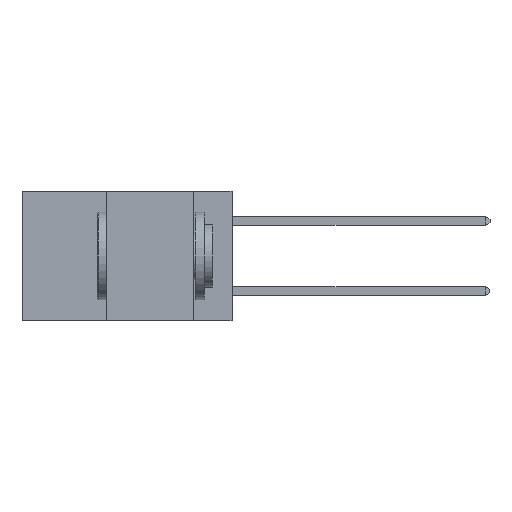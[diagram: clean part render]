
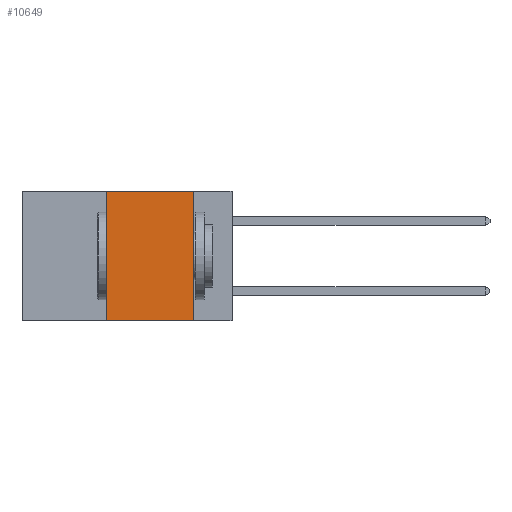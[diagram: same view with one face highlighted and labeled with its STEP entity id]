
A CAD part, left-side view. The second image highlights one B-rep face of the part: STEP entity #10649.
In plain terms, the highlighted planar face has unit normal (-1, 0, 0).
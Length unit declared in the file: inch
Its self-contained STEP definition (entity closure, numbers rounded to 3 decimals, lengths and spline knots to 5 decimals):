
#204 = EDGE_LOOP ( 'NONE', ( #6877, #7581, #6577, #3862 ) ) ;
#587 = VERTEX_POINT ( 'NONE', #3094 ) ;
#622 = VECTOR ( 'NONE', #2187, 39.37008 ) ;
#633 = FACE_OUTER_BOUND ( 'NONE', #204, .T. ) ;
#963 = EDGE_CURVE ( 'NONE', #6944, #587, #4065, .T. ) ;
#1502 = CARTESIAN_POINT ( 'NONE',  ( 0., 0.36, 0. ) ) ;
#1844 = CARTESIAN_POINT ( 'NONE',  ( 0., 0.6, 0. ) ) ;
#1886 = CARTESIAN_POINT ( 'NONE',  ( 0., 0.11, 0. ) ) ;
#2187 = DIRECTION ( 'NONE',  ( 0., 0., -1. ) ) ;
#2209 = CARTESIAN_POINT ( 'NONE',  ( 0., 0.11, 0. ) ) ;
#2719 = EDGE_CURVE ( 'NONE', #6666, #587, #5091, .T. ) ;
#2733 = DIRECTION ( 'NONE',  ( 0., 0., 1. ) ) ;
#3077 = AXIS2_PLACEMENT_3D ( 'NONE', #1844, #9297, #4334 ) ;
#3094 = CARTESIAN_POINT ( 'NONE',  ( 0., 0.11, -0.37 ) ) ;
#3494 = PLANE ( 'NONE',  #3077 ) ;
#3534 = CARTESIAN_POINT ( 'NONE',  ( 0., 0.36, 0. ) ) ;
#3862 = ORIENTED_EDGE ( 'NONE', *, *, #963, .T. ) ;
#4065 = LINE ( 'NONE', #6530, #10682 ) ;
#4091 = VECTOR ( 'NONE', #2733, 39.37008 ) ;
#4119 = DIRECTION ( 'NONE',  ( 0., -1., 0. ) ) ;
#4334 = DIRECTION ( 'NONE',  ( 0., 0., -1. ) ) ;
#4460 = VERTEX_POINT ( 'NONE', #1502 ) ;
#5091 = LINE ( 'NONE', #2209, #622 ) ;
#6470 = DIRECTION ( 'NONE',  ( 0., -1., 0. ) ) ;
#6530 = CARTESIAN_POINT ( 'NONE',  ( 0., 0.6, -0.37 ) ) ;
#6577 = ORIENTED_EDGE ( 'NONE', *, *, #7743, .F. ) ;
#6666 = VERTEX_POINT ( 'NONE', #1886 ) ;
#6877 = ORIENTED_EDGE ( 'NONE', *, *, #2719, .F. ) ;
#6944 = VERTEX_POINT ( 'NONE', #7144 ) ;
#7144 = CARTESIAN_POINT ( 'NONE',  ( 0., 0.36, -0.37 ) ) ;
#7581 = ORIENTED_EDGE ( 'NONE', *, *, #10512, .F. ) ;
#7743 = EDGE_CURVE ( 'NONE', #6944, #4460, #10705, .T. ) ;
#8306 = VECTOR ( 'NONE', #4119, 39.37008 ) ;
#9092 = CARTESIAN_POINT ( 'NONE',  ( 0., 0.6, 0. ) ) ;
#9297 = DIRECTION ( 'NONE',  ( 1., 0., 0. ) ) ;
#10512 = EDGE_CURVE ( 'NONE', #4460, #6666, #10532, .T. ) ;
#10532 = LINE ( 'NONE', #9092, #8306 ) ;
#10649 = ADVANCED_FACE ( 'NONE', ( #633 ), #3494, .F. ) ;
#10682 = VECTOR ( 'NONE', #6470, 39.37008 ) ;
#10705 = LINE ( 'NONE', #3534, #4091 ) ;
